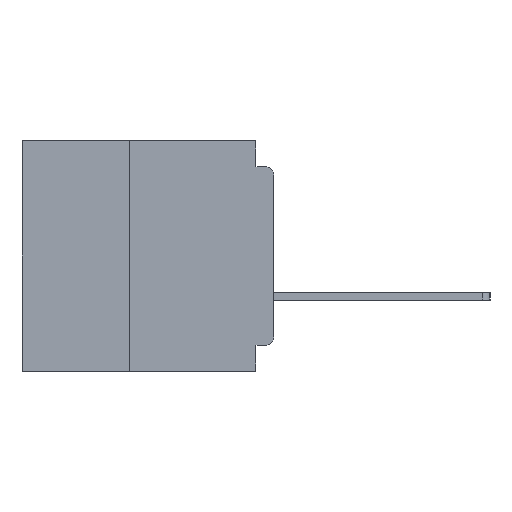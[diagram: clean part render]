
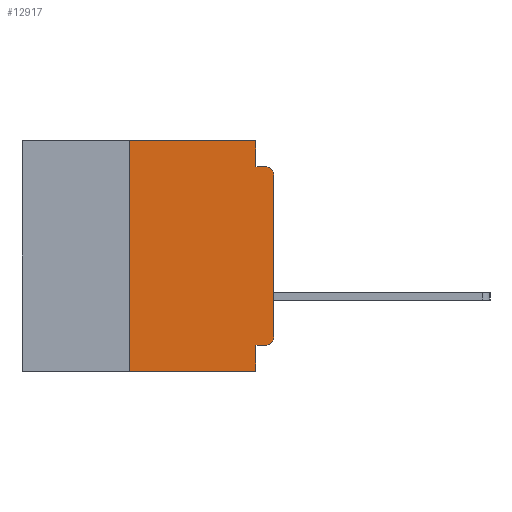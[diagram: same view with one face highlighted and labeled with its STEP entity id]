
A CAD part, left-side view. The second image highlights one B-rep face of the part: STEP entity #12917.
In plain terms, the highlighted planar face has unit normal (-1, 0, 0).
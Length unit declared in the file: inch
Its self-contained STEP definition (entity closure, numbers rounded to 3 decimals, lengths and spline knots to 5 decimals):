
#623 = DIRECTION ( 'NONE',  ( -1., 0., 0. ) ) ;
#1645 = VECTOR ( 'NONE', #14553, 39.37008 ) ;
#2666 = VERTEX_POINT ( 'NONE', #45700 ) ;
#4755 = EDGE_CURVE ( 'NONE', #48674, #13627, #51391, .T. ) ;
#5077 = VECTOR ( 'NONE', #40548, 39.37008 ) ;
#5314 = CIRCLE ( 'NONE', #20739, 0.015 ) ;
#5383 = LINE ( 'NONE', #14543, #27051 ) ;
#6003 = CARTESIAN_POINT ( 'NONE',  ( 0., 0.25, -0.4 ) ) ;
#6496 = ORIENTED_EDGE ( 'NONE', *, *, #10689, .T. ) ;
#7392 = LINE ( 'NONE', #17984, #27758 ) ;
#7674 = CARTESIAN_POINT ( 'NONE',  ( 0., 0.25, 0. ) ) ;
#8165 = CARTESIAN_POINT ( 'NONE',  ( 0., 0.015, -0.06 ) ) ;
#8400 = VECTOR ( 'NONE', #34295, 39.37008 ) ;
#8425 = LINE ( 'NONE', #17506, #50170 ) ;
#9524 = DIRECTION ( 'NONE',  ( 0., 1., 0. ) ) ;
#10027 = CARTESIAN_POINT ( 'NONE',  ( 0., 0.031, -0.4 ) ) ;
#10379 = VERTEX_POINT ( 'NONE', #6003 ) ;
#10689 = EDGE_CURVE ( 'NONE', #2666, #32938, #28814, .T. ) ;
#12258 = DIRECTION ( 'NONE',  ( 0., 0., -1. ) ) ;
#12917 = ADVANCED_FACE ( 'NONE', ( #41180 ), #14804, .F. ) ;
#13627 = VERTEX_POINT ( 'NONE', #51447 ) ;
#14543 = CARTESIAN_POINT ( 'NONE',  ( 0., 0.437, -0.4 ) ) ;
#14553 = DIRECTION ( 'NONE',  ( 0., 0., 1. ) ) ;
#14804 = PLANE ( 'NONE',  #51547 ) ;
#15138 = LINE ( 'NONE', #34736, #1645 ) ;
#15737 = EDGE_CURVE ( 'NONE', #10379, #13627, #5383, .T. ) ;
#16185 = VERTEX_POINT ( 'NONE', #49984 ) ;
#17506 = CARTESIAN_POINT ( 'NONE',  ( 0., 0., -0.355 ) ) ;
#17984 = CARTESIAN_POINT ( 'NONE',  ( 0., 0.437, 0. ) ) ;
#18041 = AXIS2_PLACEMENT_3D ( 'NONE', #8165, #36508, #12258 ) ;
#18446 = CARTESIAN_POINT ( 'NONE',  ( 0., 0.015, -0.355 ) ) ;
#18645 = ORIENTED_EDGE ( 'NONE', *, *, #21199, .F. ) ;
#19024 = CARTESIAN_POINT ( 'NONE',  ( 0., 0.031, -0.355 ) ) ;
#19392 = CARTESIAN_POINT ( 'NONE',  ( 0., 0.031, 0. ) ) ;
#20315 = ORIENTED_EDGE ( 'NONE', *, *, #15737, .T. ) ;
#20739 = AXIS2_PLACEMENT_3D ( 'NONE', #25110, #623, #29212 ) ;
#20942 = ORIENTED_EDGE ( 'NONE', *, *, #37438, .F. ) ;
#21196 = ORIENTED_EDGE ( 'NONE', *, *, #23281, .T. ) ;
#21199 = EDGE_CURVE ( 'NONE', #10379, #45053, #35982, .T. ) ;
#21355 = ORIENTED_EDGE ( 'NONE', *, *, #49615, .T. ) ;
#22072 = DIRECTION ( 'NONE',  ( 0., -1., 0. ) ) ;
#22977 = DIRECTION ( 'NONE',  ( 0., 0., -1. ) ) ;
#23281 = EDGE_CURVE ( 'NONE', #16185, #2666, #15138, .T. ) ;
#25110 = CARTESIAN_POINT ( 'NONE',  ( 0., 0.015, -0.34 ) ) ;
#25123 = VERTEX_POINT ( 'NONE', #50848 ) ;
#25423 = CARTESIAN_POINT ( 'NONE',  ( 0., 0.031, -0.045 ) ) ;
#26420 = VECTOR ( 'NONE', #47641, 39.37008 ) ;
#26752 = LINE ( 'NONE', #28330, #5077 ) ;
#27000 = EDGE_CURVE ( 'NONE', #36204, #48674, #8425, .T. ) ;
#27051 = VECTOR ( 'NONE', #51065, 39.37008 ) ;
#27363 = CARTESIAN_POINT ( 'NONE',  ( 0., 0.015, -0.045 ) ) ;
#27758 = VECTOR ( 'NONE', #22072, 39.37008 ) ;
#28330 = CARTESIAN_POINT ( 'NONE',  ( 0., 0., -0.045 ) ) ;
#28814 = CIRCLE ( 'NONE', #18041, 0.015 ) ;
#29212 = DIRECTION ( 'NONE',  ( 0., 0., -1. ) ) ;
#30922 = CARTESIAN_POINT ( 'NONE',  ( 0., 0.437, 0. ) ) ;
#31323 = ORIENTED_EDGE ( 'NONE', *, *, #4755, .F. ) ;
#32938 = VERTEX_POINT ( 'NONE', #27363 ) ;
#33541 = DIRECTION ( 'NONE',  ( 0., 0., 1. ) ) ;
#34295 = DIRECTION ( 'NONE',  ( 0., 0., -1. ) ) ;
#34713 = VECTOR ( 'NONE', #33541, 39.37008 ) ;
#34736 = CARTESIAN_POINT ( 'NONE',  ( 0., 0., 0. ) ) ;
#35982 = LINE ( 'NONE', #49375, #34713 ) ;
#36204 = VERTEX_POINT ( 'NONE', #18446 ) ;
#36508 = DIRECTION ( 'NONE',  ( -1., 0., 0. ) ) ;
#36880 = ORIENTED_EDGE ( 'NONE', *, *, #48508, .F. ) ;
#37160 = LINE ( 'NONE', #19392, #26420 ) ;
#37438 = EDGE_CURVE ( 'NONE', #25123, #45293, #37160, .T. ) ;
#40494 = ORIENTED_EDGE ( 'NONE', *, *, #27000, .F. ) ;
#40548 = DIRECTION ( 'NONE',  ( 0., -1., 0. ) ) ;
#41180 = FACE_OUTER_BOUND ( 'NONE', #42791, .T. ) ;
#41959 = ORIENTED_EDGE ( 'NONE', *, *, #51302, .F. ) ;
#42791 = EDGE_LOOP ( 'NONE', ( #21196, #6496, #41959, #20942, #36880, #18645, #20315, #31323, #40494, #21355 ) ) ;
#45053 = VERTEX_POINT ( 'NONE', #7674 ) ;
#45293 = VERTEX_POINT ( 'NONE', #25423 ) ;
#45700 = CARTESIAN_POINT ( 'NONE',  ( 0., 0., -0.06 ) ) ;
#47131 = DIRECTION ( 'NONE',  ( 1., 0., 0. ) ) ;
#47641 = DIRECTION ( 'NONE',  ( 0., 0., -1. ) ) ;
#48508 = EDGE_CURVE ( 'NONE', #45053, #25123, #7392, .T. ) ;
#48674 = VERTEX_POINT ( 'NONE', #19024 ) ;
#49375 = CARTESIAN_POINT ( 'NONE',  ( 0., 0.25, -0.4 ) ) ;
#49615 = EDGE_CURVE ( 'NONE', #36204, #16185, #5314, .T. ) ;
#49984 = CARTESIAN_POINT ( 'NONE',  ( 0., 0., -0.34 ) ) ;
#50170 = VECTOR ( 'NONE', #9524, 39.37008 ) ;
#50848 = CARTESIAN_POINT ( 'NONE',  ( 0., 0.031, 0. ) ) ;
#51065 = DIRECTION ( 'NONE',  ( 0., -1., 0. ) ) ;
#51302 = EDGE_CURVE ( 'NONE', #45293, #32938, #26752, .T. ) ;
#51391 = LINE ( 'NONE', #10027, #8400 ) ;
#51447 = CARTESIAN_POINT ( 'NONE',  ( 0., 0.031, -0.4 ) ) ;
#51547 = AXIS2_PLACEMENT_3D ( 'NONE', #30922, #47131, #22977 ) ;
